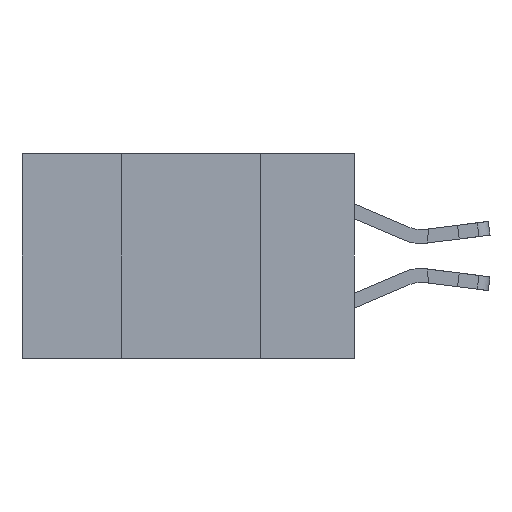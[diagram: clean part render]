
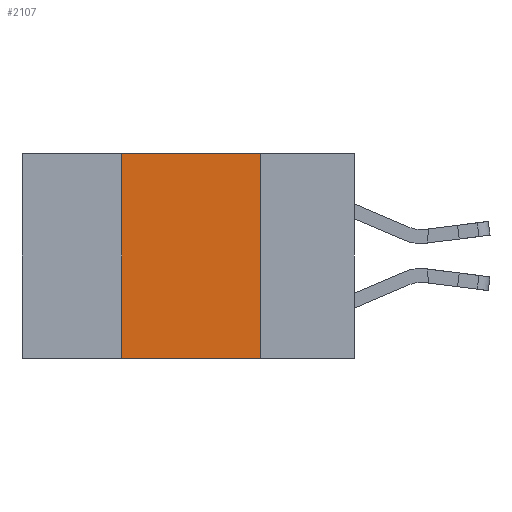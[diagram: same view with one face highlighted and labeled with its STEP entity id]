
A CAD part, left-side view. The second image highlights one B-rep face of the part: STEP entity #2107.
In plain terms, the highlighted planar face has unit normal (-1, 0, 0).
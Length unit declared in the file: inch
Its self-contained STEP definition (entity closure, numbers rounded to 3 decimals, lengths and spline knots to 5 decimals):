
#521 = CARTESIAN_POINT ( 'NONE',  ( 0., 0.42, 0. ) ) ;
#914 = CARTESIAN_POINT ( 'NONE',  ( 0., 0.42, -0.37 ) ) ;
#1149 = DIRECTION ( 'NONE',  ( 0., 0., 1. ) ) ;
#1221 = LINE ( 'NONE', #8110, #3506 ) ;
#1389 = VECTOR ( 'NONE', #1149, 39.37008 ) ;
#1497 = CARTESIAN_POINT ( 'NONE',  ( 0., 0.17, 0. ) ) ;
#1854 = PLANE ( 'NONE',  #18077 ) ;
#2107 = ADVANCED_FACE ( 'NONE', ( #3428 ), #1854, .F. ) ;
#2628 = VERTEX_POINT ( 'NONE', #1497 ) ;
#2709 = LINE ( 'NONE', #9610, #6099 ) ;
#3428 = FACE_OUTER_BOUND ( 'NONE', #21855, .T. ) ;
#3506 = VECTOR ( 'NONE', #20232, 39.37008 ) ;
#4355 = ORIENTED_EDGE ( 'NONE', *, *, #12097, .T. ) ;
#6063 = EDGE_CURVE ( 'NONE', #2628, #13594, #1221, .T. ) ;
#6099 = VECTOR ( 'NONE', #9727, 39.37008 ) ;
#8110 = CARTESIAN_POINT ( 'NONE',  ( 0., 0.17, -0.37 ) ) ;
#9431 = CARTESIAN_POINT ( 'NONE',  ( 0., 0.17, -0.37 ) ) ;
#9610 = CARTESIAN_POINT ( 'NONE',  ( 0., 0.6, -0.37 ) ) ;
#9727 = DIRECTION ( 'NONE',  ( 0., -1., 0. ) ) ;
#11066 = DIRECTION ( 'NONE',  ( 0., -1., 0. ) ) ;
#11219 = EDGE_CURVE ( 'NONE', #15971, #13674, #13225, .T. ) ;
#11521 = EDGE_CURVE ( 'NONE', #13674, #2628, #17749, .T. ) ;
#12097 = EDGE_CURVE ( 'NONE', #15971, #13594, #2709, .T. ) ;
#12244 = CARTESIAN_POINT ( 'NONE',  ( 0., 0.6, 0. ) ) ;
#12266 = CARTESIAN_POINT ( 'NONE',  ( 0., 0.42, -0.37 ) ) ;
#13225 = LINE ( 'NONE', #914, #1389 ) ;
#13594 = VERTEX_POINT ( 'NONE', #9431 ) ;
#13674 = VERTEX_POINT ( 'NONE', #521 ) ;
#14433 = ORIENTED_EDGE ( 'NONE', *, *, #11219, .F. ) ;
#15971 = VERTEX_POINT ( 'NONE', #12266 ) ;
#16708 = ORIENTED_EDGE ( 'NONE', *, *, #11521, .F. ) ;
#17749 = LINE ( 'NONE', #17856, #22019 ) ;
#17856 = CARTESIAN_POINT ( 'NONE',  ( 0., 0.6, 0. ) ) ;
#17954 = ORIENTED_EDGE ( 'NONE', *, *, #6063, .F. ) ;
#18077 = AXIS2_PLACEMENT_3D ( 'NONE', #12244, #20867, #19155 ) ;
#19155 = DIRECTION ( 'NONE',  ( 0., 0., -1. ) ) ;
#20232 = DIRECTION ( 'NONE',  ( 0., 0., -1. ) ) ;
#20867 = DIRECTION ( 'NONE',  ( 1., 0., 0. ) ) ;
#21855 = EDGE_LOOP ( 'NONE', ( #17954, #16708, #14433, #4355 ) ) ;
#22019 = VECTOR ( 'NONE', #11066, 39.37008 ) ;
